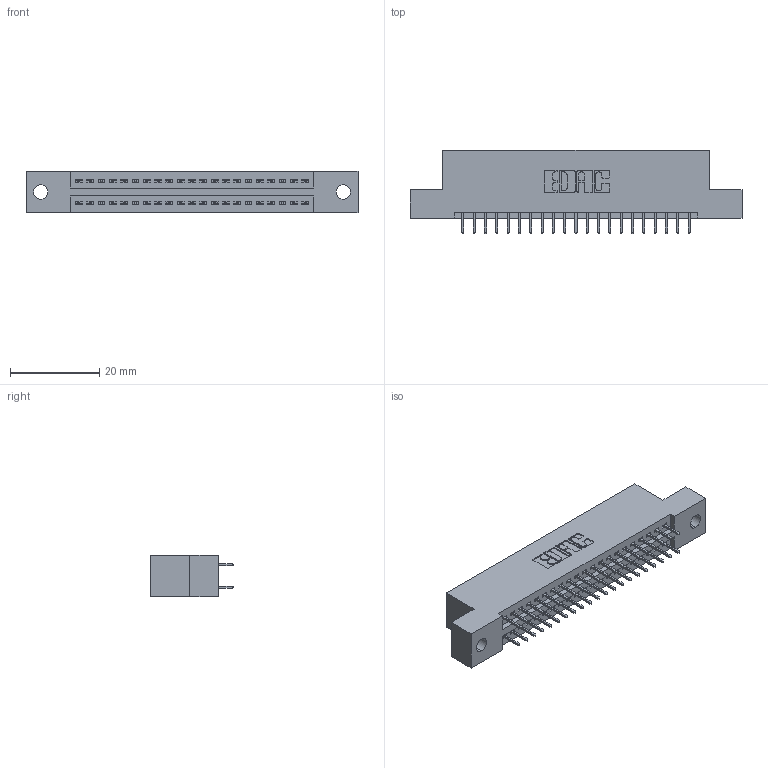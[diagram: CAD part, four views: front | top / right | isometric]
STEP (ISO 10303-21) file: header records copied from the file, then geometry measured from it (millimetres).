
FILE_DESCRIPTION (( 'STEP AP203' ), '1' );
FILE_NAME ('845-042-525-202.STEP', '2020-09-23T05:38:52', ( '' ), ( '' ), 'SwSTEP 2.0', 'SolidWorks 2020', '' );
FILE_SCHEMA (( 'CONFIG_CONTROL_DESIGN' ));
Length unit declared in the file: inch
Products named in the file (3): 845-042-525-202; 845 Part_Flush Mounting Lugs - 0.128 Dia; 345-292-001_345-293-125
Assembly tree (43 placements, depth 2):
  845-042-525-202
    845 Part_Flush Mounting Lugs - 0.128 Dia
    345-292-001_345-293-125  x42
Bounding box: 74.55 x 18.72 x 9.4 mm (x, y, z)
Volume: 6941 mm3; surface area: 9372.2 mm2
Topology: 43 solids, 43 shells, 2394 faces, 6767 edges, 4342 vertices
Faces by surface type: plane 1718, cylinder 676
Entity records: 19381 total; most frequent: CARTESIAN_POINT 3268, ORIENTED_EDGE 3202, DIRECTION 2909, EDGE_CURVE 1601, LINE 1389, VECTOR 1389, VERTEX_POINT 1062, AXIS2_PLACEMENT_3D 760
